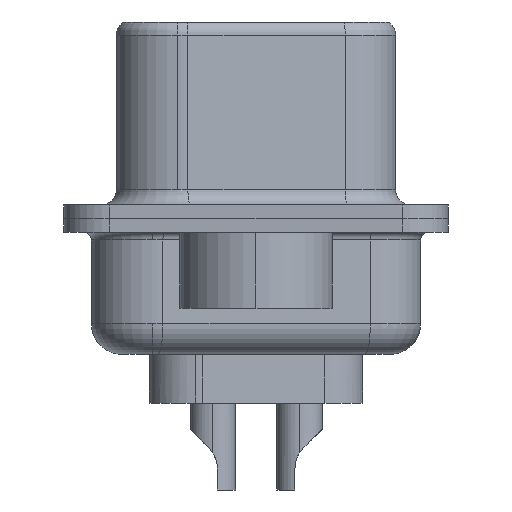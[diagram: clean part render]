
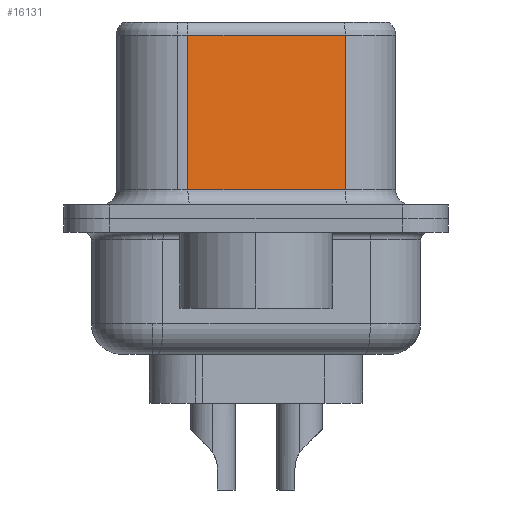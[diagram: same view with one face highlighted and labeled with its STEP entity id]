
A CAD part, left-side view. The second image highlights one B-rep face of the part: STEP entity #16131.
In plain terms, the highlighted planar face has unit normal (-0.985, -0.174, 0).
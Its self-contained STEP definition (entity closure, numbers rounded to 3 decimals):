
#560 = ORIENTED_EDGE ( 'NONE', *, *, #14703, .F. ) ;
#1119 = CARTESIAN_POINT ( 'NONE',  ( 4.575, -2.927, 6.52 ) ) ;
#1568 = ORIENTED_EDGE ( 'NONE', *, *, #16586, .T. ) ;
#1585 = CARTESIAN_POINT ( 'NONE',  ( 4.575, -2.927, 0.95 ) ) ;
#1709 = DIRECTION ( 'NONE',  ( 0.985, 0.174, 0. ) ) ;
#3329 = VERTEX_POINT ( 'NONE', #4964 ) ;
#4044 = EDGE_CURVE ( 'NONE', #6156, #13690, #17610, .T. ) ;
#4964 = CARTESIAN_POINT ( 'NONE',  ( 3.665, 2.233, 0.95 ) ) ;
#5837 = VERTEX_POINT ( 'NONE', #5935 ) ;
#5935 = CARTESIAN_POINT ( 'NONE',  ( 4.575, -2.927, 0.95 ) ) ;
#6156 = VERTEX_POINT ( 'NONE', #12386 ) ;
#6178 = VECTOR ( 'NONE', #18743, 1000. ) ;
#6200 = VECTOR ( 'NONE', #9181, 1000. ) ;
#6857 = EDGE_LOOP ( 'NONE', ( #560, #18548, #10940, #1568 ) ) ;
#6950 = LINE ( 'NONE', #1119, #11003 ) ;
#7517 = PLANE ( 'NONE',  #11042 ) ;
#7839 = LINE ( 'NONE', #11748, #6200 ) ;
#8374 = EDGE_CURVE ( 'NONE', #13690, #3329, #7839, .T. ) ;
#9049 = FACE_OUTER_BOUND ( 'NONE', #6857, .T. ) ;
#9181 = DIRECTION ( 'NONE',  ( 0., 0., -1. ) ) ;
#10070 = LINE ( 'NONE', #1585, #6178 ) ;
#10279 = DIRECTION ( 'NONE',  ( -0.174, 0.985, 0. ) ) ;
#10940 = ORIENTED_EDGE ( 'NONE', *, *, #8374, .T. ) ;
#11003 = VECTOR ( 'NONE', #11052, 1000. ) ;
#11042 = AXIS2_PLACEMENT_3D ( 'NONE', #12935, #1709, #15999 ) ;
#11052 = DIRECTION ( 'NONE',  ( 0., 0., -1. ) ) ;
#11232 = VECTOR ( 'NONE', #10279, 1000. ) ;
#11748 = CARTESIAN_POINT ( 'NONE',  ( 3.665, 2.233, 6.52 ) ) ;
#12386 = CARTESIAN_POINT ( 'NONE',  ( 4.575, -2.927, 6.02 ) ) ;
#12935 = CARTESIAN_POINT ( 'NONE',  ( 4.575, -2.927, 6.52 ) ) ;
#13690 = VERTEX_POINT ( 'NONE', #13854 ) ;
#13854 = CARTESIAN_POINT ( 'NONE',  ( 3.665, 2.233, 6.02 ) ) ;
#14646 = CARTESIAN_POINT ( 'NONE',  ( 4.575, -2.927, 6.02 ) ) ;
#14703 = EDGE_CURVE ( 'NONE', #6156, #5837, #6950, .T. ) ;
#15999 = DIRECTION ( 'NONE',  ( -0.174, 0.985, 0. ) ) ;
#16131 = ADVANCED_FACE ( 'NONE', ( #9049 ), #7517, .F. ) ;
#16586 = EDGE_CURVE ( 'NONE', #3329, #5837, #10070, .T. ) ;
#17610 = LINE ( 'NONE', #14646, #11232 ) ;
#18548 = ORIENTED_EDGE ( 'NONE', *, *, #4044, .T. ) ;
#18743 = DIRECTION ( 'NONE',  ( 0.174, -0.985, 0. ) ) ;
